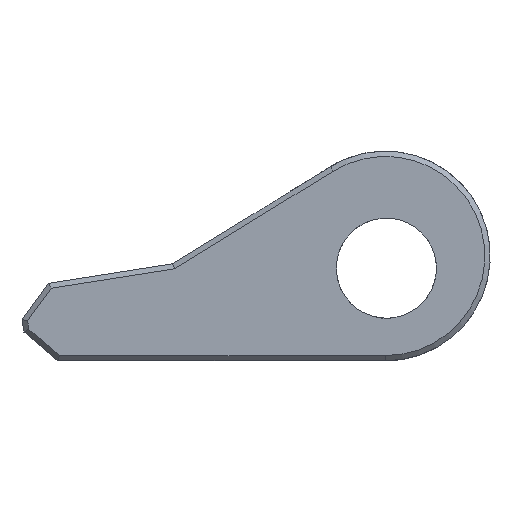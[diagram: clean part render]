
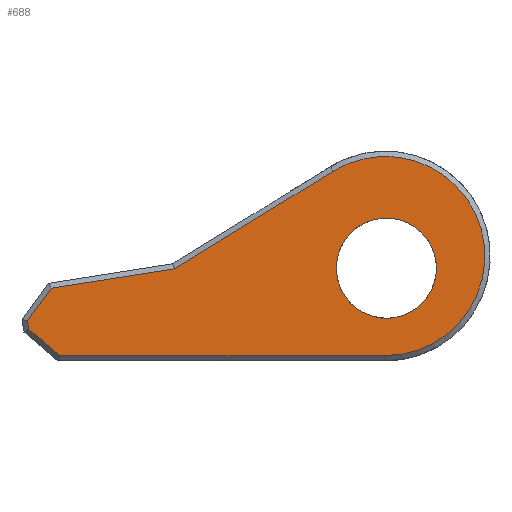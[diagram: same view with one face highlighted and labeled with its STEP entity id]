
A CAD part, front view. The second image highlights one B-rep face of the part: STEP entity #688.
In plain terms, the highlighted planar face has unit normal (0, -1, 0).
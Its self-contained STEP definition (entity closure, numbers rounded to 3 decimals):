
#16=FACE_BOUND('',#117,.T.);
#35=CIRCLE('',#717,4.75);
#42=CIRCLE('',#752,9.45);
#78=FACE_OUTER_BOUND('',#116,.T.);
#116=EDGE_LOOP('',(#612,#613,#614,#615,#616,#617,#618));
#117=EDGE_LOOP('',(#619));
#180=LINE('',#1145,#255);
#184=LINE('',#1153,#259);
#187=LINE('',#1158,#262);
#189=LINE('',#1162,#264);
#192=LINE('',#1170,#267);
#194=LINE('',#1173,#269);
#255=VECTOR('',#906,10.);
#259=VECTOR('',#912,10.);
#262=VECTOR('',#917,10.);
#264=VECTOR('',#921,10.);
#267=VECTOR('',#930,10.);
#269=VECTOR('',#934,10.);
#295=VERTEX_POINT('',#998);
#324=VERTEX_POINT('',#1143);
#325=VERTEX_POINT('',#1144);
#328=VERTEX_POINT('',#1152);
#329=VERTEX_POINT('',#1157);
#330=VERTEX_POINT('',#1161);
#331=VERTEX_POINT('',#1165);
#332=VERTEX_POINT('',#1169);
#357=EDGE_CURVE('',#295,#295,#35,.T.);
#411=EDGE_CURVE('',#324,#325,#180,.T.);
#415=EDGE_CURVE('',#325,#328,#184,.T.);
#418=EDGE_CURVE('',#328,#329,#187,.T.);
#420=EDGE_CURVE('',#329,#330,#189,.T.);
#423=EDGE_CURVE('',#330,#331,#42,.T.);
#424=EDGE_CURVE('',#331,#332,#192,.T.);
#426=EDGE_CURVE('',#332,#324,#194,.T.);
#612=ORIENTED_EDGE('',*,*,#411,.F.);
#613=ORIENTED_EDGE('',*,*,#426,.F.);
#614=ORIENTED_EDGE('',*,*,#424,.F.);
#615=ORIENTED_EDGE('',*,*,#423,.F.);
#616=ORIENTED_EDGE('',*,*,#420,.F.);
#617=ORIENTED_EDGE('',*,*,#418,.F.);
#618=ORIENTED_EDGE('',*,*,#415,.F.);
#619=ORIENTED_EDGE('',*,*,#357,.T.);
#651=PLANE('',#757);
#688=ADVANCED_FACE('',(#78,#16),#651,.F.);
#717=AXIS2_PLACEMENT_3D('',#999,#803,#804);
#752=AXIS2_PLACEMENT_3D('',#1167,#926,#927);
#757=AXIS2_PLACEMENT_3D('',#1179,#942,#943);
#803=DIRECTION('center_axis',(0.,1.,0.));
#804=DIRECTION('ref_axis',(0.426,0.,0.905));
#906=DIRECTION('',(-0.155,0.,0.988));
#912=DIRECTION('',(0.589,0.,0.808));
#917=DIRECTION('',(0.988,0.,0.155));
#921=DIRECTION('',(0.852,0.,0.524));
#926=DIRECTION('center_axis',(0.,1.,0.));
#927=DIRECTION('ref_axis',(-0.155,0.,0.988));
#930=DIRECTION('',(-1.,0.,0.));
#934=DIRECTION('',(-0.76,0.,0.65));
#942=DIRECTION('center_axis',(0.,1.,0.));
#943=DIRECTION('ref_axis',(0.155,0.,-0.988));
#998=CARTESIAN_POINT('',(-17.143,57.508,4.498));
#999=CARTESIAN_POINT('Origin',(-15.12,57.508,8.796));
#1143=CARTESIAN_POINT('',(-49.049,57.508,2.995));
#1144=CARTESIAN_POINT('',(-49.176,57.508,3.799));
#1145=CARTESIAN_POINT('',(-49.098,57.508,3.307));
#1152=CARTESIAN_POINT('',(-46.923,57.508,6.894));
#1153=CARTESIAN_POINT('',(-44.077,57.508,10.803));
#1157=CARTESIAN_POINT('',(-35.239,57.508,8.733));
#1158=CARTESIAN_POINT('',(-39.471,57.508,8.067));
#1161=CARTESIAN_POINT('',(-20.169,57.508,18.));
#1162=CARTESIAN_POINT('',(-30.977,57.508,11.354));
#1165=CARTESIAN_POINT('',(-15.219,57.508,0.5));
#1167=CARTESIAN_POINT('Origin',(-15.219,57.508,9.95));
#1169=CARTESIAN_POINT('',(-46.131,57.508,0.5));
#1170=CARTESIAN_POINT('',(-21.887,57.508,0.5));
#1173=CARTESIAN_POINT('',(-44.037,57.508,-1.29));
#1179=CARTESIAN_POINT('Origin',(-28.555,57.508,7.851));
